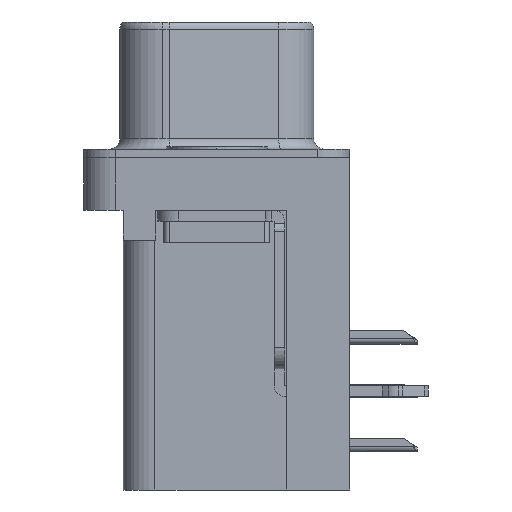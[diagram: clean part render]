
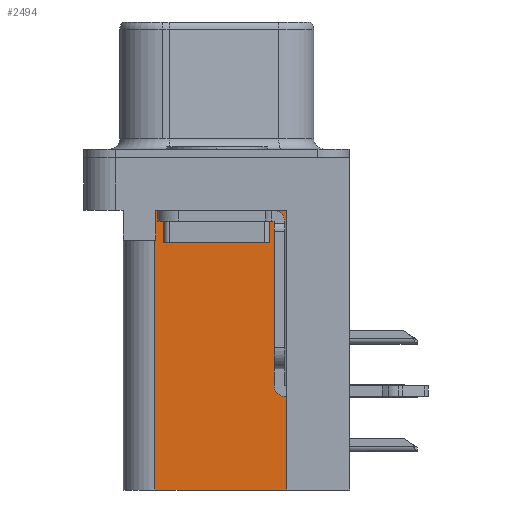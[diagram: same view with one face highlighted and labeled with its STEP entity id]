
A CAD part, left-side view. The second image highlights one B-rep face of the part: STEP entity #2494.
In plain terms, the highlighted planar face has unit normal (-1, 0, 0).
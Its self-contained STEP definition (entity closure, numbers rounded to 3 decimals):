
#494 = LINE ( 'NONE', #12922, #9141 ) ;
#2384 = DIRECTION ( 'NONE',  ( 0., 0., 1. ) ) ;
#2494 = ADVANCED_FACE ( 'NONE', ( #11845 ), #12271, .F. ) ;
#2781 = ORIENTED_EDGE ( 'NONE', *, *, #16830, .T. ) ;
#3161 = EDGE_CURVE ( 'NONE', #6026, #12691, #494, .T. ) ;
#3214 = VECTOR ( 'NONE', #13585, 1000. ) ;
#3835 = EDGE_LOOP ( 'NONE', ( #14908, #2781, #17654, #21451, #13639, #17189 ) ) ;
#4544 = EDGE_CURVE ( 'NONE', #12691, #6229, #17875, .T. ) ;
#4759 = CARTESIAN_POINT ( 'NONE',  ( 3.765, -3.295, -15.7 ) ) ;
#5770 = CARTESIAN_POINT ( 'NONE',  ( 3.765, 2.925, -15.7 ) ) ;
#6026 = VERTEX_POINT ( 'NONE', #9188 ) ;
#6229 = VERTEX_POINT ( 'NONE', #9849 ) ;
#6249 = CARTESIAN_POINT ( 'NONE',  ( 3.765, -3.295, -2.5 ) ) ;
#6498 = DIRECTION ( 'NONE',  ( 0., 1., 0. ) ) ;
#6814 = CARTESIAN_POINT ( 'NONE',  ( 3.765, 2.925, -15.7 ) ) ;
#7670 = VECTOR ( 'NONE', #6498, 1000. ) ;
#7783 = CARTESIAN_POINT ( 'NONE',  ( 3.765, -3.295, -15.7 ) ) ;
#7992 = LINE ( 'NONE', #5770, #16998 ) ;
#8179 = EDGE_CURVE ( 'NONE', #20393, #8324, #8235, .T. ) ;
#8210 = LINE ( 'NONE', #4759, #7670 ) ;
#8235 = LINE ( 'NONE', #17966, #21326 ) ;
#8324 = VERTEX_POINT ( 'NONE', #20102 ) ;
#8689 = EDGE_CURVE ( 'NONE', #19021, #8324, #7992, .T. ) ;
#9141 = VECTOR ( 'NONE', #10929, 1000. ) ;
#9188 = CARTESIAN_POINT ( 'NONE',  ( 3.765, -3.295, -15.7 ) ) ;
#9509 = DIRECTION ( 'NONE',  ( 0., 1., 0. ) ) ;
#9849 = CARTESIAN_POINT ( 'NONE',  ( 3.765, 2.895, -2.5 ) ) ;
#10480 = DIRECTION ( 'NONE',  ( 0., 1., 0. ) ) ;
#10929 = DIRECTION ( 'NONE',  ( 0., 0., 1. ) ) ;
#11845 = FACE_OUTER_BOUND ( 'NONE', #3835, .T. ) ;
#12271 = PLANE ( 'NONE',  #18716 ) ;
#12691 = VERTEX_POINT ( 'NONE', #16248 ) ;
#12845 = VECTOR ( 'NONE', #10480, 1000. ) ;
#12922 = CARTESIAN_POINT ( 'NONE',  ( 3.765, -3.295, -15.7 ) ) ;
#13585 = DIRECTION ( 'NONE',  ( 0., 0., -1. ) ) ;
#13639 = ORIENTED_EDGE ( 'NONE', *, *, #18238, .F. ) ;
#14908 = ORIENTED_EDGE ( 'NONE', *, *, #4544, .T. ) ;
#15454 = DIRECTION ( 'NONE',  ( 1., 0., 0. ) ) ;
#16248 = CARTESIAN_POINT ( 'NONE',  ( 3.765, -3.295, -2.5 ) ) ;
#16830 = EDGE_CURVE ( 'NONE', #6229, #20393, #20823, .T. ) ;
#16998 = VECTOR ( 'NONE', #2384, 1000. ) ;
#17189 = ORIENTED_EDGE ( 'NONE', *, *, #3161, .T. ) ;
#17654 = ORIENTED_EDGE ( 'NONE', *, *, #8179, .T. ) ;
#17875 = LINE ( 'NONE', #6249, #12845 ) ;
#17966 = CARTESIAN_POINT ( 'NONE',  ( 3.765, 0., -3.9 ) ) ;
#18238 = EDGE_CURVE ( 'NONE', #6026, #19021, #8210, .T. ) ;
#18716 = AXIS2_PLACEMENT_3D ( 'NONE', #7783, #15454, #19250 ) ;
#19021 = VERTEX_POINT ( 'NONE', #6814 ) ;
#19216 = CARTESIAN_POINT ( 'NONE',  ( 3.765, 2.895, -3.9 ) ) ;
#19250 = DIRECTION ( 'NONE',  ( 0., 0., -1. ) ) ;
#20102 = CARTESIAN_POINT ( 'NONE',  ( 3.765, 2.925, -3.9 ) ) ;
#20393 = VERTEX_POINT ( 'NONE', #19216 ) ;
#20536 = CARTESIAN_POINT ( 'NONE',  ( 3.765, 2.895, -3.9 ) ) ;
#20823 = LINE ( 'NONE', #20536, #3214 ) ;
#21326 = VECTOR ( 'NONE', #9509, 1000. ) ;
#21451 = ORIENTED_EDGE ( 'NONE', *, *, #8689, .F. ) ;
